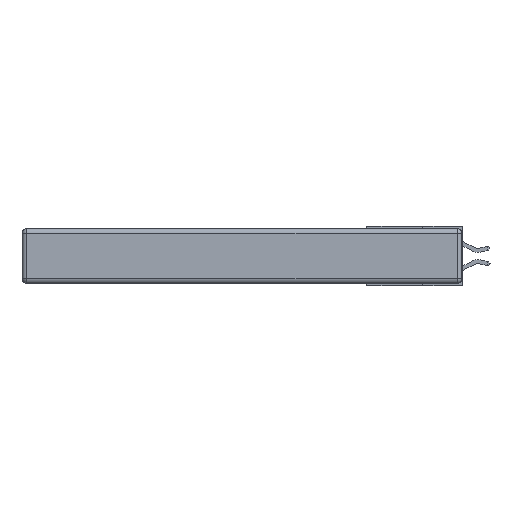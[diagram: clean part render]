
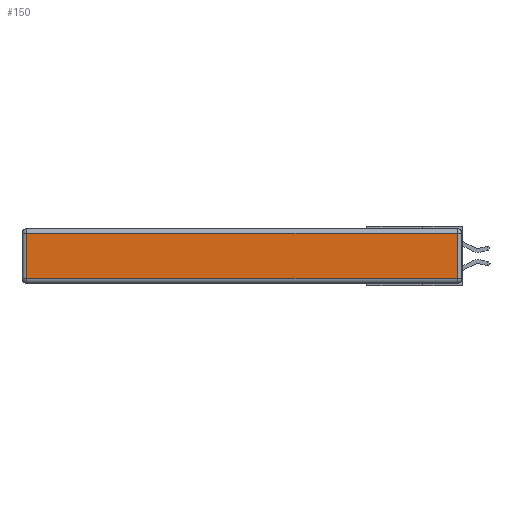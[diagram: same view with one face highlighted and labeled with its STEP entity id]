
A CAD part, left-side view. The second image highlights one B-rep face of the part: STEP entity #150.
In plain terms, the highlighted planar face has unit normal (-1, 0, 0).
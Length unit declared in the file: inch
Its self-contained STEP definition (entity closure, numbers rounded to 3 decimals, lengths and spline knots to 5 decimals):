
#150 = ADVANCED_FACE ( 'NONE', ( #13111 ), #6029, .T. ) ;
#1060 = EDGE_CURVE ( 'NONE', #7681, #2916, #16256, .T. ) ;
#1199 = ORIENTED_EDGE ( 'NONE', *, *, #14908, .T. ) ;
#2245 = CARTESIAN_POINT ( 'NONE',  ( 0., 0.03, -0.313 ) ) ;
#2342 = VECTOR ( 'NONE', #9030, 39.37008 ) ;
#2355 = EDGE_CURVE ( 'NONE', #11232, #5890, #10987, .T. ) ;
#2382 = CARTESIAN_POINT ( 'NONE',  ( 0., 0., -0.313 ) ) ;
#2916 = VERTEX_POINT ( 'NONE', #12160 ) ;
#4322 = VECTOR ( 'NONE', #15316, 39.37008 ) ;
#4804 = CARTESIAN_POINT ( 'NONE',  ( 0., 2.72, -0.313 ) ) ;
#5193 = LINE ( 'NONE', #16798, #2342 ) ;
#5276 = DIRECTION ( 'NONE',  ( 0., -1., 0. ) ) ;
#5890 = VERTEX_POINT ( 'NONE', #2245 ) ;
#6029 = PLANE ( 'NONE',  #16394 ) ;
#7681 = VERTEX_POINT ( 'NONE', #14250 ) ;
#8461 = DIRECTION ( 'NONE',  ( 0., 0., 1. ) ) ;
#8636 = CARTESIAN_POINT ( 'NONE',  ( 0., 0., -0.343 ) ) ;
#8806 = EDGE_CURVE ( 'NONE', #2916, #11232, #5193, .T. ) ;
#9030 = DIRECTION ( 'NONE',  ( 0., 0., -1. ) ) ;
#9376 = VECTOR ( 'NONE', #16459, 39.37008 ) ;
#10858 = ORIENTED_EDGE ( 'NONE', *, *, #1060, .T. ) ;
#10987 = LINE ( 'NONE', #2382, #13047 ) ;
#11232 = VERTEX_POINT ( 'NONE', #4804 ) ;
#12160 = CARTESIAN_POINT ( 'NONE',  ( 0., 2.72, -0.03 ) ) ;
#12476 = CARTESIAN_POINT ( 'NONE',  ( 0., 2.75, -0.03 ) ) ;
#13047 = VECTOR ( 'NONE', #5276, 39.37008 ) ;
#13111 = FACE_OUTER_BOUND ( 'NONE', #16367, .T. ) ;
#13668 = LINE ( 'NONE', #15373, #4322 ) ;
#14250 = CARTESIAN_POINT ( 'NONE',  ( 0., 0.03, -0.03 ) ) ;
#14908 = EDGE_CURVE ( 'NONE', #5890, #7681, #13668, .T. ) ;
#15129 = ORIENTED_EDGE ( 'NONE', *, *, #2355, .T. ) ;
#15255 = ORIENTED_EDGE ( 'NONE', *, *, #8806, .T. ) ;
#15316 = DIRECTION ( 'NONE',  ( 0., 0., 1. ) ) ;
#15373 = CARTESIAN_POINT ( 'NONE',  ( 0., 0.03, -0.343 ) ) ;
#16256 = LINE ( 'NONE', #12476, #9376 ) ;
#16367 = EDGE_LOOP ( 'NONE', ( #15129, #1199, #10858, #15255 ) ) ;
#16390 = DIRECTION ( 'NONE',  ( -1., 0., 0. ) ) ;
#16394 = AXIS2_PLACEMENT_3D ( 'NONE', #8636, #16390, #8461 ) ;
#16459 = DIRECTION ( 'NONE',  ( 0., 1., 0. ) ) ;
#16798 = CARTESIAN_POINT ( 'NONE',  ( 0., 2.72, -0.343 ) ) ;
